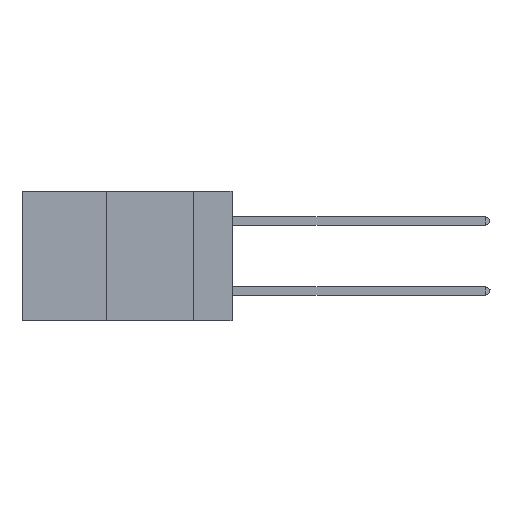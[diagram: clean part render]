
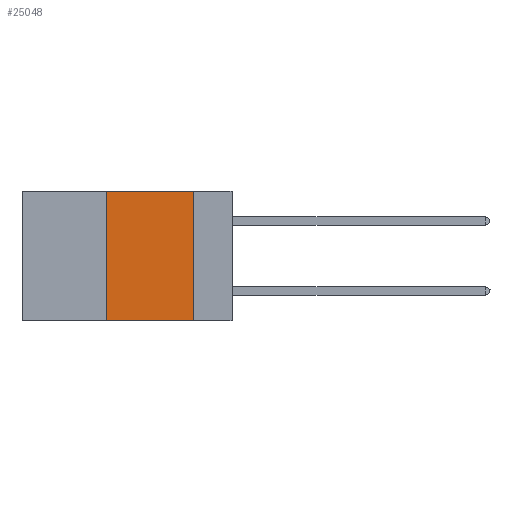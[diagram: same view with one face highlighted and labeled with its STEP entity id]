
A CAD part, left-side view. The second image highlights one B-rep face of the part: STEP entity #25048.
In plain terms, the highlighted planar face has unit normal (-1, 0, 0).
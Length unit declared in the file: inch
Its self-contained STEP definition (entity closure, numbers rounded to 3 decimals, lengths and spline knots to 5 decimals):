
#593 = DIRECTION ( 'NONE',  ( 0., -1., 0. ) ) ;
#1220 = ORIENTED_EDGE ( 'NONE', *, *, #22925, .F. ) ;
#1259 = CARTESIAN_POINT ( 'NONE',  ( 0., 0.6, 0. ) ) ;
#2831 = VERTEX_POINT ( 'NONE', #24826 ) ;
#3013 = CARTESIAN_POINT ( 'NONE',  ( 0., 0.11, 0. ) ) ;
#3161 = VECTOR ( 'NONE', #28353, 39.37008 ) ;
#3496 = VECTOR ( 'NONE', #593, 39.37008 ) ;
#3776 = AXIS2_PLACEMENT_3D ( 'NONE', #6475, #11686, #13975 ) ;
#3890 = PLANE ( 'NONE',  #3776 ) ;
#5148 = EDGE_CURVE ( 'NONE', #22716, #28458, #12979, .T. ) ;
#5510 = CARTESIAN_POINT ( 'NONE',  ( 0., 0.36, -0.37 ) ) ;
#6475 = CARTESIAN_POINT ( 'NONE',  ( 0., 0.6, 0. ) ) ;
#7342 = VECTOR ( 'NONE', #15686, 39.37008 ) ;
#7885 = DIRECTION ( 'NONE',  ( 0., 0., -1. ) ) ;
#9565 = VERTEX_POINT ( 'NONE', #3013 ) ;
#11514 = EDGE_LOOP ( 'NONE', ( #20590, #1220, #21415, #23899 ) ) ;
#11686 = DIRECTION ( 'NONE',  ( 1., 0., 0. ) ) ;
#12979 = LINE ( 'NONE', #22952, #3496 ) ;
#13975 = DIRECTION ( 'NONE',  ( 0., 0., -1. ) ) ;
#15686 = DIRECTION ( 'NONE',  ( 0., 0., 1. ) ) ;
#17823 = LINE ( 'NONE', #18310, #7342 ) ;
#18310 = CARTESIAN_POINT ( 'NONE',  ( 0., 0.36, 0. ) ) ;
#19006 = EDGE_CURVE ( 'NONE', #9565, #28458, #19185, .T. ) ;
#19185 = LINE ( 'NONE', #29117, #27324 ) ;
#20590 = ORIENTED_EDGE ( 'NONE', *, *, #19006, .F. ) ;
#21415 = ORIENTED_EDGE ( 'NONE', *, *, #23401, .F. ) ;
#21561 = CARTESIAN_POINT ( 'NONE',  ( 0., 0.11, -0.37 ) ) ;
#22716 = VERTEX_POINT ( 'NONE', #5510 ) ;
#22925 = EDGE_CURVE ( 'NONE', #2831, #9565, #26228, .T. ) ;
#22952 = CARTESIAN_POINT ( 'NONE',  ( 0., 0.6, -0.37 ) ) ;
#23401 = EDGE_CURVE ( 'NONE', #22716, #2831, #17823, .T. ) ;
#23899 = ORIENTED_EDGE ( 'NONE', *, *, #5148, .T. ) ;
#24826 = CARTESIAN_POINT ( 'NONE',  ( 0., 0.36, 0. ) ) ;
#25048 = ADVANCED_FACE ( 'NONE', ( #26717 ), #3890, .F. ) ;
#26228 = LINE ( 'NONE', #1259, #3161 ) ;
#26717 = FACE_OUTER_BOUND ( 'NONE', #11514, .T. ) ;
#27324 = VECTOR ( 'NONE', #7885, 39.37008 ) ;
#28353 = DIRECTION ( 'NONE',  ( 0., -1., 0. ) ) ;
#28458 = VERTEX_POINT ( 'NONE', #21561 ) ;
#29117 = CARTESIAN_POINT ( 'NONE',  ( 0., 0.11, 0. ) ) ;
